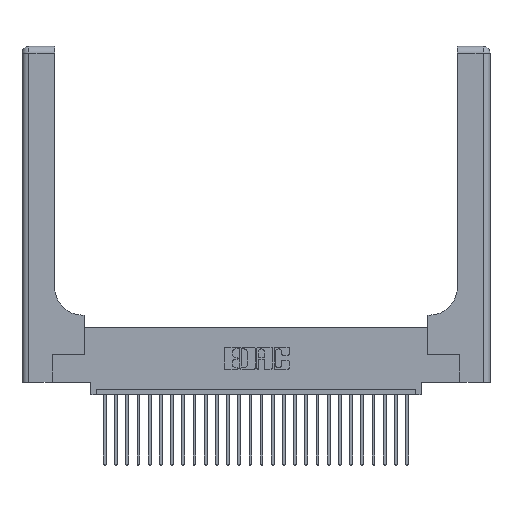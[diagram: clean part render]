
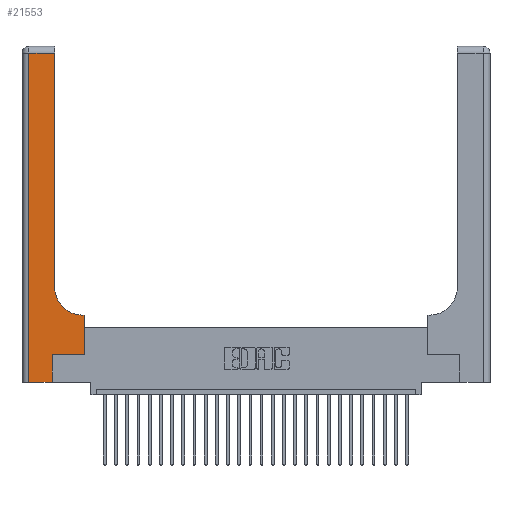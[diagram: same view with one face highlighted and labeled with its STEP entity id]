
A CAD part, top view. The second image highlights one B-rep face of the part: STEP entity #21553.
In plain terms, the highlighted planar face has unit normal (0, 0, 1).
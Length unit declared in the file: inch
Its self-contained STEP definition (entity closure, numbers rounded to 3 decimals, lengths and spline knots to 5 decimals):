
#612 = DIRECTION ( 'NONE',  ( 1., 0., 0. ) ) ;
#784 = CARTESIAN_POINT ( 'NONE',  ( 0.269, 0., 0.37 ) ) ;
#1713 = VERTEX_POINT ( 'NONE', #27863 ) ;
#1917 = ORIENTED_EDGE ( 'NONE', *, *, #19666, .T. ) ;
#2044 = ORIENTED_EDGE ( 'NONE', *, *, #11400, .T. ) ;
#2306 = VERTEX_POINT ( 'NONE', #14182 ) ;
#2566 = ORIENTED_EDGE ( 'NONE', *, *, #6334, .T. ) ;
#2737 = LINE ( 'NONE', #10721, #10998 ) ;
#3869 = DIRECTION ( 'NONE',  ( 1., 0., 0. ) ) ;
#4116 = EDGE_LOOP ( 'NONE', ( #28318, #12226, #2044, #15017, #24275, #1917, #6110, #24682, #2566 ) ) ;
#4122 = VERTEX_POINT ( 'NONE', #11377 ) ;
#4526 = LINE ( 'NONE', #6861, #8990 ) ;
#4655 = VECTOR ( 'NONE', #24293, 39.37008 ) ;
#5249 = CARTESIAN_POINT ( 'NONE',  ( 0.5415, 0.6, 0.37 ) ) ;
#6110 = ORIENTED_EDGE ( 'NONE', *, *, #18317, .T. ) ;
#6334 = EDGE_CURVE ( 'NONE', #10939, #1713, #20277, .T. ) ;
#6552 = DIRECTION ( 'NONE',  ( -1., 0., 0. ) ) ;
#6861 = CARTESIAN_POINT ( 'NONE',  ( 0.5585, 0.25, 0.37 ) ) ;
#7427 = DIRECTION ( 'NONE',  ( 0., 1., 0. ) ) ;
#7711 = CARTESIAN_POINT ( 'NONE',  ( 0., 2.94, 0.37 ) ) ;
#8588 = AXIS2_PLACEMENT_3D ( 'NONE', #10648, #23972, #612 ) ;
#8747 = CARTESIAN_POINT ( 'NONE',  ( 0.5585, 0.6, 0.37 ) ) ;
#8778 = VERTEX_POINT ( 'NONE', #25815 ) ;
#8814 = LINE ( 'NONE', #7711, #18090 ) ;
#8887 = CARTESIAN_POINT ( 'NONE',  ( 0.269, 0.25, 0.37 ) ) ;
#8990 = VECTOR ( 'NONE', #11502, 39.37008 ) ;
#9506 = LINE ( 'NONE', #12416, #20485 ) ;
#9545 = FACE_OUTER_BOUND ( 'NONE', #4116, .T. ) ;
#10534 = LINE ( 'NONE', #784, #10869 ) ;
#10648 = CARTESIAN_POINT ( 'NONE',  ( 0.5415, 0.85, 0.37 ) ) ;
#10721 = CARTESIAN_POINT ( 'NONE',  ( 0., 0., 0.37 ) ) ;
#10869 = VECTOR ( 'NONE', #7427, 39.37008 ) ;
#10939 = VERTEX_POINT ( 'NONE', #5249 ) ;
#10998 = VECTOR ( 'NONE', #3869, 39.37008 ) ;
#11377 = CARTESIAN_POINT ( 'NONE',  ( 0.269, 0., 0.37 ) ) ;
#11400 = EDGE_CURVE ( 'NONE', #18006, #2306, #9506, .T. ) ;
#11401 = VERTEX_POINT ( 'NONE', #23299 ) ;
#11502 = DIRECTION ( 'NONE',  ( 0., 1., 0. ) ) ;
#11718 = VECTOR ( 'NONE', #13594, 39.37008 ) ;
#11906 = EDGE_CURVE ( 'NONE', #18155, #10939, #28298, .T. ) ;
#12226 = ORIENTED_EDGE ( 'NONE', *, *, #21960, .T. ) ;
#12416 = CARTESIAN_POINT ( 'NONE',  ( 0.06, 3., 0.37 ) ) ;
#13594 = DIRECTION ( 'NONE',  ( 1., 0., 0. ) ) ;
#14182 = CARTESIAN_POINT ( 'NONE',  ( 0.06, 0., 0.37 ) ) ;
#14954 = VERTEX_POINT ( 'NONE', #25767 ) ;
#15017 = ORIENTED_EDGE ( 'NONE', *, *, #20584, .T. ) ;
#15330 = VECTOR ( 'NONE', #26374, 39.37008 ) ;
#16685 = AXIS2_PLACEMENT_3D ( 'NONE', #26171, #26080, #6552 ) ;
#17710 = LINE ( 'NONE', #22321, #15330 ) ;
#18006 = VERTEX_POINT ( 'NONE', #20951 ) ;
#18090 = VECTOR ( 'NONE', #20863, 39.37008 ) ;
#18155 = VERTEX_POINT ( 'NONE', #8747 ) ;
#18317 = EDGE_CURVE ( 'NONE', #8778, #18155, #4526, .T. ) ;
#19666 = EDGE_CURVE ( 'NONE', #11401, #8778, #23717, .T. ) ;
#20277 = CIRCLE ( 'NONE', #8588, 0.25 ) ;
#20485 = VECTOR ( 'NONE', #21120, 39.37008 ) ;
#20584 = EDGE_CURVE ( 'NONE', #2306, #4122, #2737, .T. ) ;
#20863 = DIRECTION ( 'NONE',  ( -1., 0., 0. ) ) ;
#20951 = CARTESIAN_POINT ( 'NONE',  ( 0.06, 2.94, 0.37 ) ) ;
#21120 = DIRECTION ( 'NONE',  ( 0., -1., 0. ) ) ;
#21553 = ADVANCED_FACE ( 'NONE', ( #9545 ), #23995, .F. ) ;
#21960 = EDGE_CURVE ( 'NONE', #14954, #18006, #8814, .T. ) ;
#22321 = CARTESIAN_POINT ( 'NONE',  ( 0.2915, 3., 0.37 ) ) ;
#22921 = EDGE_CURVE ( 'NONE', #4122, #11401, #10534, .T. ) ;
#23299 = CARTESIAN_POINT ( 'NONE',  ( 0.269, 0.25, 0.37 ) ) ;
#23717 = LINE ( 'NONE', #8887, #11718 ) ;
#23972 = DIRECTION ( 'NONE',  ( 0., 0., -1. ) ) ;
#23995 = PLANE ( 'NONE',  #16685 ) ;
#24275 = ORIENTED_EDGE ( 'NONE', *, *, #22921, .T. ) ;
#24293 = DIRECTION ( 'NONE',  ( -1., 0., 0. ) ) ;
#24682 = ORIENTED_EDGE ( 'NONE', *, *, #11906, .T. ) ;
#25767 = CARTESIAN_POINT ( 'NONE',  ( 0.2915, 2.94, 0.37 ) ) ;
#25815 = CARTESIAN_POINT ( 'NONE',  ( 0.5585, 0.25, 0.37 ) ) ;
#25858 = EDGE_CURVE ( 'NONE', #1713, #14954, #17710, .T. ) ;
#26080 = DIRECTION ( 'NONE',  ( 0., 0., -1. ) ) ;
#26171 = CARTESIAN_POINT ( 'NONE',  ( 0., 3., 0.37 ) ) ;
#26374 = DIRECTION ( 'NONE',  ( 0., 1., 0. ) ) ;
#27814 = CARTESIAN_POINT ( 'NONE',  ( 0.2915, 0.6, 0.37 ) ) ;
#27863 = CARTESIAN_POINT ( 'NONE',  ( 0.2915, 0.85, 0.37 ) ) ;
#28298 = LINE ( 'NONE', #27814, #4655 ) ;
#28318 = ORIENTED_EDGE ( 'NONE', *, *, #25858, .T. ) ;
